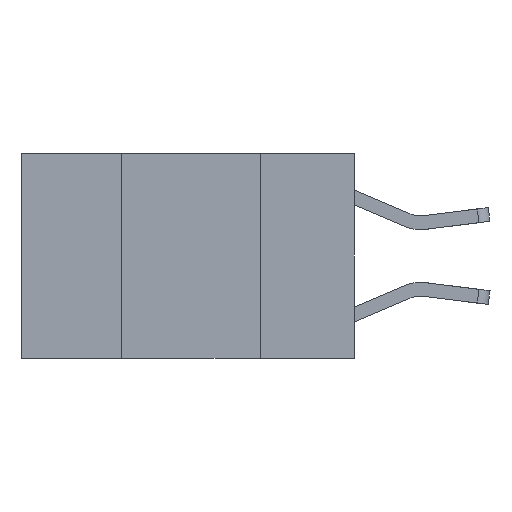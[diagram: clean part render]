
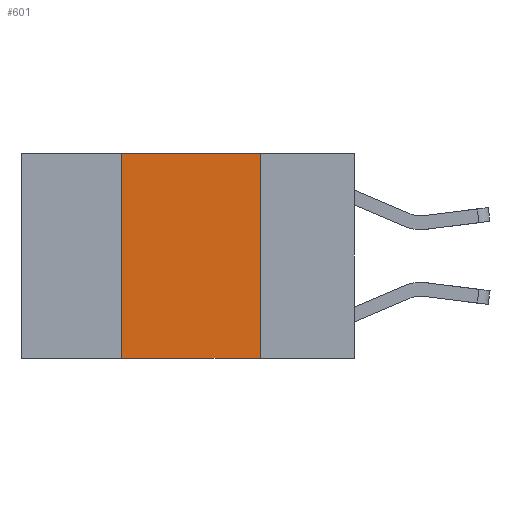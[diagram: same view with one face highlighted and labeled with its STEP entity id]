
A CAD part, left-side view. The second image highlights one B-rep face of the part: STEP entity #601.
In plain terms, the highlighted planar face has unit normal (-1, 0, 0).
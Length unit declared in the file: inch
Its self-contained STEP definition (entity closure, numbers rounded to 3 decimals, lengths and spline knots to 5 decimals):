
#427 = LINE ( 'NONE', #784, #5276 ) ;
#534 = VERTEX_POINT ( 'NONE', #9969 ) ;
#586 = DIRECTION ( 'NONE',  ( 0., 0., -1. ) ) ;
#601 = ADVANCED_FACE ( 'NONE', ( #4620 ), #5405, .F. ) ;
#784 = CARTESIAN_POINT ( 'NONE',  ( 0., 0.6, 0. ) ) ;
#1382 = VERTEX_POINT ( 'NONE', #11506 ) ;
#1755 = DIRECTION ( 'NONE',  ( 0., -1., 0. ) ) ;
#2038 = CARTESIAN_POINT ( 'NONE',  ( 0., 0.42, -0.37 ) ) ;
#2338 = DIRECTION ( 'NONE',  ( 0., -1., 0. ) ) ;
#2487 = VECTOR ( 'NONE', #2338, 39.37008 ) ;
#2900 = LINE ( 'NONE', #9328, #10328 ) ;
#2946 = EDGE_CURVE ( 'NONE', #4507, #1382, #9270, .T. ) ;
#3116 = DIRECTION ( 'NONE',  ( 0., 0., 1. ) ) ;
#3703 = AXIS2_PLACEMENT_3D ( 'NONE', #4430, #6378, #586 ) ;
#4077 = ORIENTED_EDGE ( 'NONE', *, *, #6466, .F. ) ;
#4430 = CARTESIAN_POINT ( 'NONE',  ( 0., 0.6, 0. ) ) ;
#4507 = VERTEX_POINT ( 'NONE', #2038 ) ;
#4620 = FACE_OUTER_BOUND ( 'NONE', #7505, .T. ) ;
#5018 = ORIENTED_EDGE ( 'NONE', *, *, #5385, .T. ) ;
#5276 = VECTOR ( 'NONE', #1755, 39.37008 ) ;
#5384 = LINE ( 'NONE', #8132, #2487 ) ;
#5385 = EDGE_CURVE ( 'NONE', #4507, #534, #5384, .T. ) ;
#5405 = PLANE ( 'NONE',  #3703 ) ;
#6028 = CARTESIAN_POINT ( 'NONE',  ( 0., 0.42, 0. ) ) ;
#6378 = DIRECTION ( 'NONE',  ( 1., 0., 0. ) ) ;
#6466 = EDGE_CURVE ( 'NONE', #7236, #534, #2900, .T. ) ;
#6705 = VECTOR ( 'NONE', #3116, 39.37008 ) ;
#7236 = VERTEX_POINT ( 'NONE', #9479 ) ;
#7505 = EDGE_LOOP ( 'NONE', ( #4077, #9851, #12405, #5018 ) ) ;
#8132 = CARTESIAN_POINT ( 'NONE',  ( 0., 0.6, -0.37 ) ) ;
#8342 = DIRECTION ( 'NONE',  ( 0., 0., -1. ) ) ;
#9270 = LINE ( 'NONE', #6028, #6705 ) ;
#9328 = CARTESIAN_POINT ( 'NONE',  ( 0., 0.17, 0. ) ) ;
#9479 = CARTESIAN_POINT ( 'NONE',  ( 0., 0.17, 0. ) ) ;
#9851 = ORIENTED_EDGE ( 'NONE', *, *, #10085, .F. ) ;
#9969 = CARTESIAN_POINT ( 'NONE',  ( 0., 0.17, -0.37 ) ) ;
#10085 = EDGE_CURVE ( 'NONE', #1382, #7236, #427, .T. ) ;
#10328 = VECTOR ( 'NONE', #8342, 39.37008 ) ;
#11506 = CARTESIAN_POINT ( 'NONE',  ( 0., 0.42, 0. ) ) ;
#12405 = ORIENTED_EDGE ( 'NONE', *, *, #2946, .F. ) ;
